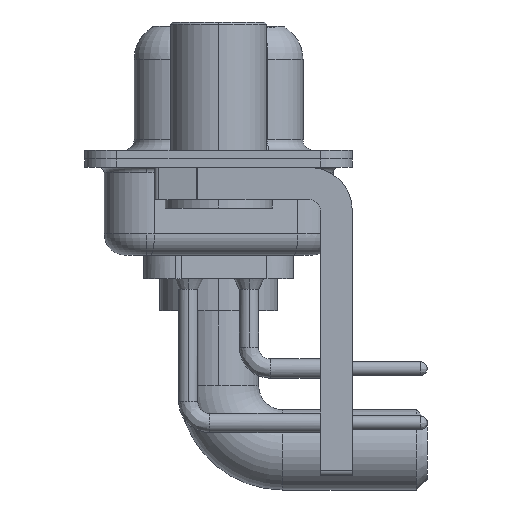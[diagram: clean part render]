
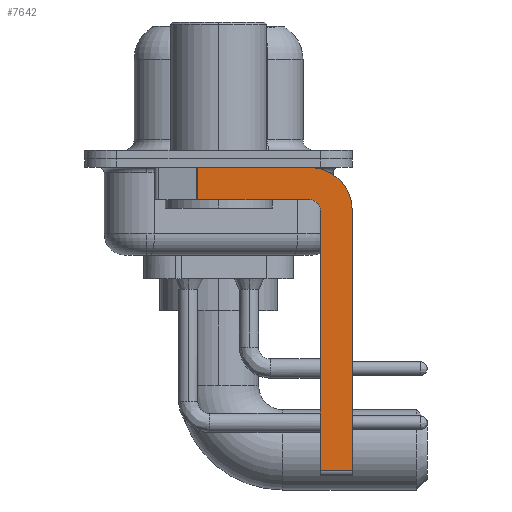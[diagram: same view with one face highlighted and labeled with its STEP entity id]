
A CAD part, left-side view. The second image highlights one B-rep face of the part: STEP entity #7642.
In plain terms, the highlighted planar face has unit normal (-1, 0, 0).
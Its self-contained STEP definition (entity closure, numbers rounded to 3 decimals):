
#886 = VECTOR ( 'NONE', #16314, 1000. ) ;
#1100 = VECTOR ( 'NONE', #8716, 1000. ) ;
#1180 = VERTEX_POINT ( 'NONE', #20372 ) ;
#1286 = DIRECTION ( 'NONE',  ( 1., 0., 0. ) ) ;
#1551 = DIRECTION ( 'NONE',  ( -1., 0., 0. ) ) ;
#1605 = CARTESIAN_POINT ( 'NONE',  ( -2.9, -4.25, -2.4 ) ) ;
#1893 = EDGE_CURVE ( 'NONE', #7830, #16902, #8493, .T. ) ;
#1969 = ORIENTED_EDGE ( 'NONE', *, *, #10139, .F. ) ;
#1983 = CARTESIAN_POINT ( 'NONE',  ( -2.9, -4.25, -1.9 ) ) ;
#2117 = ORIENTED_EDGE ( 'NONE', *, *, #15567, .F. ) ;
#2224 = VECTOR ( 'NONE', #9989, 1000. ) ;
#3842 = EDGE_LOOP ( 'NONE', ( #5114, #12198, #1969, #4152, #12096, #10554, #18980, #2117 ) ) ;
#4152 = ORIENTED_EDGE ( 'NONE', *, *, #16658, .F. ) ;
#4607 = CARTESIAN_POINT ( 'NONE',  ( -2.9, -4.25, -1.9 ) ) ;
#5114 = ORIENTED_EDGE ( 'NONE', *, *, #13420, .F. ) ;
#5166 = LINE ( 'NONE', #18120, #18942 ) ;
#5838 = CARTESIAN_POINT ( 'NONE',  ( -2.9, 0.978, -1.9 ) ) ;
#6244 = CARTESIAN_POINT ( 'NONE',  ( -2.9, -4.75, -14.55 ) ) ;
#6306 = VERTEX_POINT ( 'NONE', #11050 ) ;
#6500 = EDGE_CURVE ( 'NONE', #7830, #17182, #19620, .T. ) ;
#6741 = CIRCLE ( 'NONE', #18360, 0.5 ) ;
#7109 = PLANE ( 'NONE',  #15927 ) ;
#7210 = FACE_OUTER_BOUND ( 'NONE', #3842, .T. ) ;
#7642 = ADVANCED_FACE ( 'NONE', ( #7210 ), #7109, .F. ) ;
#7830 = VERTEX_POINT ( 'NONE', #6244 ) ;
#8100 = DIRECTION ( 'NONE',  ( 0., 0., 1. ) ) ;
#8493 = LINE ( 'NONE', #14705, #886 ) ;
#8716 = DIRECTION ( 'NONE',  ( 0., 0., -1. ) ) ;
#9650 = CARTESIAN_POINT ( 'NONE',  ( -2.9, -4.25, -14.55 ) ) ;
#9767 = CIRCLE ( 'NONE', #10812, 2. ) ;
#9989 = DIRECTION ( 'NONE',  ( 0., 0., -1. ) ) ;
#10139 = EDGE_CURVE ( 'NONE', #19059, #18205, #19290, .T. ) ;
#10192 = DIRECTION ( 'NONE',  ( 0., -1., 0. ) ) ;
#10554 = ORIENTED_EDGE ( 'NONE', *, *, #6500, .T. ) ;
#10630 = DIRECTION ( 'NONE',  ( 1., 0., 0. ) ) ;
#10812 = AXIS2_PLACEMENT_3D ( 'NONE', #1605, #1286, #17779 ) ;
#11050 = CARTESIAN_POINT ( 'NONE',  ( -2.9, -6.25, -2.4 ) ) ;
#11135 = DIRECTION ( 'NONE',  ( 0., 1., 0. ) ) ;
#11613 = VERTEX_POINT ( 'NONE', #13647 ) ;
#11682 = EDGE_CURVE ( 'NONE', #1180, #18205, #13962, .T. ) ;
#11895 = CARTESIAN_POINT ( 'NONE',  ( -2.9, -6.25, -14.55 ) ) ;
#12096 = ORIENTED_EDGE ( 'NONE', *, *, #1893, .F. ) ;
#12198 = ORIENTED_EDGE ( 'NONE', *, *, #11682, .T. ) ;
#12855 = DIRECTION ( 'NONE',  ( 0., -1., 0. ) ) ;
#13198 = LINE ( 'NONE', #19745, #2224 ) ;
#13420 = EDGE_CURVE ( 'NONE', #1180, #11613, #5166, .T. ) ;
#13647 = CARTESIAN_POINT ( 'NONE',  ( -2.9, -4.25, -0.4 ) ) ;
#13734 = DIRECTION ( 'NONE',  ( 0., 0., -1. ) ) ;
#13962 = LINE ( 'NONE', #5838, #1100 ) ;
#14705 = CARTESIAN_POINT ( 'NONE',  ( -2.9, -4.75, -14.8 ) ) ;
#15567 = EDGE_CURVE ( 'NONE', #11613, #6306, #9767, .T. ) ;
#15927 = AXIS2_PLACEMENT_3D ( 'NONE', #18783, #10630, #13734 ) ;
#16086 = CARTESIAN_POINT ( 'NONE',  ( -2.9, 0.978, -1.9 ) ) ;
#16215 = CARTESIAN_POINT ( 'NONE',  ( -2.9, -4.25, -2.4 ) ) ;
#16314 = DIRECTION ( 'NONE',  ( 0., 0., 1. ) ) ;
#16658 = EDGE_CURVE ( 'NONE', #16902, #19059, #6741, .T. ) ;
#16902 = VERTEX_POINT ( 'NONE', #19108 ) ;
#17045 = EDGE_CURVE ( 'NONE', #6306, #17182, #13198, .T. ) ;
#17182 = VERTEX_POINT ( 'NONE', #11895 ) ;
#17779 = DIRECTION ( 'NONE',  ( 0., 0., -1. ) ) ;
#18120 = CARTESIAN_POINT ( 'NONE',  ( -2.9, 3., -0.4 ) ) ;
#18205 = VERTEX_POINT ( 'NONE', #16086 ) ;
#18360 = AXIS2_PLACEMENT_3D ( 'NONE', #16215, #1551, #8100 ) ;
#18539 = VECTOR ( 'NONE', #11135, 1000. ) ;
#18620 = VECTOR ( 'NONE', #12855, 1000. ) ;
#18783 = CARTESIAN_POINT ( 'NONE',  ( -2.9, -4.25, -2.4 ) ) ;
#18942 = VECTOR ( 'NONE', #10192, 1000. ) ;
#18980 = ORIENTED_EDGE ( 'NONE', *, *, #17045, .F. ) ;
#19059 = VERTEX_POINT ( 'NONE', #1983 ) ;
#19108 = CARTESIAN_POINT ( 'NONE',  ( -2.9, -4.75, -2.4 ) ) ;
#19290 = LINE ( 'NONE', #4607, #18539 ) ;
#19620 = LINE ( 'NONE', #9650, #18620 ) ;
#19745 = CARTESIAN_POINT ( 'NONE',  ( -2.9, -6.25, -2.4 ) ) ;
#20372 = CARTESIAN_POINT ( 'NONE',  ( -2.9, 0.978, -0.4 ) ) ;
